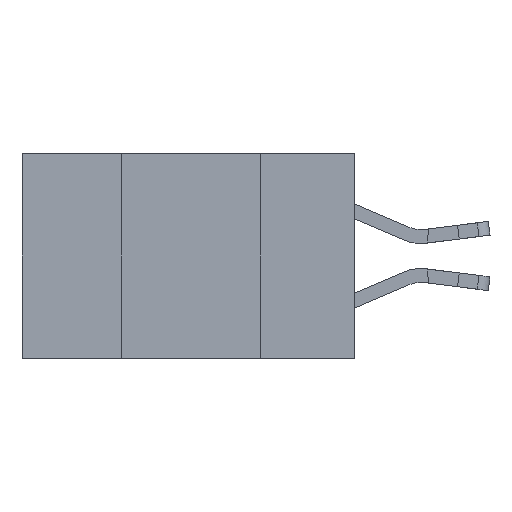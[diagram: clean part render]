
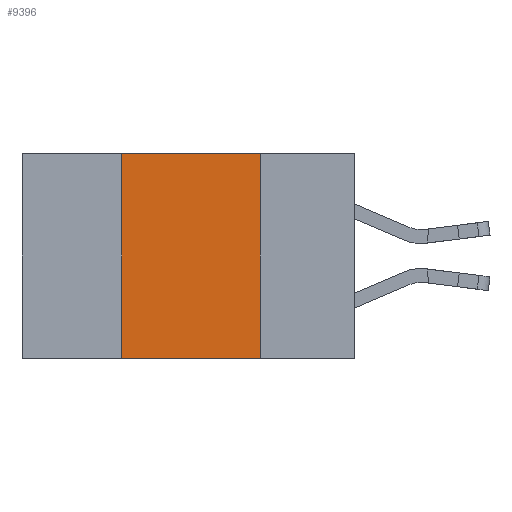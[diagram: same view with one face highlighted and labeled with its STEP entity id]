
A CAD part, left-side view. The second image highlights one B-rep face of the part: STEP entity #9396.
In plain terms, the highlighted planar face has unit normal (-1, 0, 0).
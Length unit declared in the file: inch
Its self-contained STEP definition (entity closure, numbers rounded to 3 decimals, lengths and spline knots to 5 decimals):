
#227 = ORIENTED_EDGE ( 'NONE', *, *, #1716, .F. ) ;
#242 = VERTEX_POINT ( 'NONE', #16178 ) ;
#271 = DIRECTION ( 'NONE',  ( 0., 0., -1. ) ) ;
#796 = VERTEX_POINT ( 'NONE', #13524 ) ;
#1024 = EDGE_LOOP ( 'NONE', ( #9588, #227, #9549, #9618 ) ) ;
#1606 = EDGE_CURVE ( 'NONE', #10851, #796, #6619, .T. ) ;
#1716 = EDGE_CURVE ( 'NONE', #796, #8528, #14966, .T. ) ;
#1718 = FACE_OUTER_BOUND ( 'NONE', #1024, .T. ) ;
#5338 = LINE ( 'NONE', #7212, #11684 ) ;
#6230 = CARTESIAN_POINT ( 'NONE',  ( 0., 0.42, -0.37 ) ) ;
#6619 = LINE ( 'NONE', #7488, #13193 ) ;
#7212 = CARTESIAN_POINT ( 'NONE',  ( 0., 0.17, 0. ) ) ;
#7488 = CARTESIAN_POINT ( 'NONE',  ( 0., 0.42, 0. ) ) ;
#7718 = DIRECTION ( 'NONE',  ( 1., 0., 0. ) ) ;
#8516 = DIRECTION ( 'NONE',  ( 0., 0., -1. ) ) ;
#8528 = VERTEX_POINT ( 'NONE', #13735 ) ;
#9396 = ADVANCED_FACE ( 'NONE', ( #1718 ), #10249, .F. ) ;
#9549 = ORIENTED_EDGE ( 'NONE', *, *, #1606, .F. ) ;
#9588 = ORIENTED_EDGE ( 'NONE', *, *, #14705, .F. ) ;
#9618 = ORIENTED_EDGE ( 'NONE', *, *, #13414, .T. ) ;
#10249 = PLANE ( 'NONE',  #14081 ) ;
#10851 = VERTEX_POINT ( 'NONE', #6230 ) ;
#10955 = DIRECTION ( 'NONE',  ( 0., 0., 1. ) ) ;
#11569 = DIRECTION ( 'NONE',  ( 0., -1., 0. ) ) ;
#11613 = VECTOR ( 'NONE', #11569, 39.37008 ) ;
#11684 = VECTOR ( 'NONE', #8516, 39.37008 ) ;
#12205 = DIRECTION ( 'NONE',  ( 0., -1., 0. ) ) ;
#13193 = VECTOR ( 'NONE', #10955, 39.37008 ) ;
#13414 = EDGE_CURVE ( 'NONE', #10851, #242, #15065, .T. ) ;
#13524 = CARTESIAN_POINT ( 'NONE',  ( 0., 0.42, 0. ) ) ;
#13735 = CARTESIAN_POINT ( 'NONE',  ( 0., 0.17, 0. ) ) ;
#14081 = AXIS2_PLACEMENT_3D ( 'NONE', #15308, #7718, #271 ) ;
#14280 = VECTOR ( 'NONE', #12205, 39.37008 ) ;
#14705 = EDGE_CURVE ( 'NONE', #8528, #242, #5338, .T. ) ;
#14966 = LINE ( 'NONE', #15736, #11613 ) ;
#15065 = LINE ( 'NONE', #15955, #14280 ) ;
#15308 = CARTESIAN_POINT ( 'NONE',  ( 0., 0.6, 0. ) ) ;
#15736 = CARTESIAN_POINT ( 'NONE',  ( 0., 0.6, 0. ) ) ;
#15955 = CARTESIAN_POINT ( 'NONE',  ( 0., 0.6, -0.37 ) ) ;
#16178 = CARTESIAN_POINT ( 'NONE',  ( 0., 0.17, -0.37 ) ) ;
